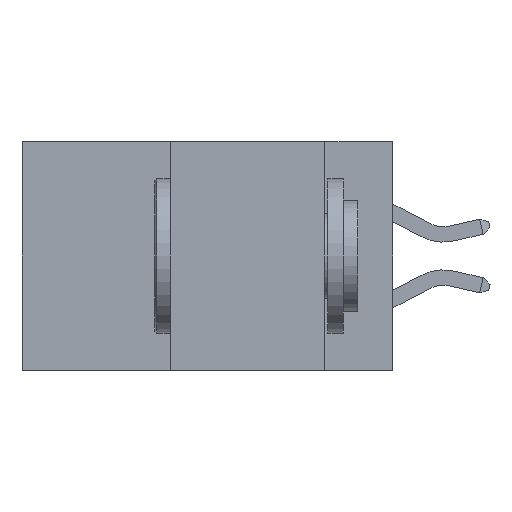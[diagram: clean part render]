
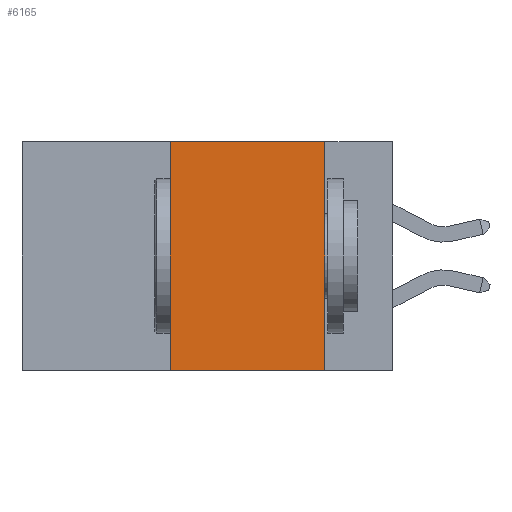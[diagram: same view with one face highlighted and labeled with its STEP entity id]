
A CAD part, left-side view. The second image highlights one B-rep face of the part: STEP entity #6165.
In plain terms, the highlighted planar face has unit normal (-1, 0, 0).
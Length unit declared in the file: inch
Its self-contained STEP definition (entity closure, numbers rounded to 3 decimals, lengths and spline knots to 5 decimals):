
#2321 = VERTEX_POINT ( 'NONE', #10326 ) ;
#2730 = AXIS2_PLACEMENT_3D ( 'NONE', #5660, #5352, #22209 ) ;
#3332 = CARTESIAN_POINT ( 'NONE',  ( 0., 0.11, 0. ) ) ;
#5352 = DIRECTION ( 'NONE',  ( 1., 0., 0. ) ) ;
#5660 = CARTESIAN_POINT ( 'NONE',  ( 0., 0.6, 0. ) ) ;
#6165 = ADVANCED_FACE ( 'NONE', ( #21445 ), #10330, .F. ) ;
#6452 = EDGE_CURVE ( 'NONE', #12743, #2321, #17380, .T. ) ;
#6535 = VERTEX_POINT ( 'NONE', #13450 ) ;
#8285 = EDGE_LOOP ( 'NONE', ( #12414, #28717, #10790, #28006 ) ) ;
#10326 = CARTESIAN_POINT ( 'NONE',  ( 0., 0.11, -0.37 ) ) ;
#10330 = PLANE ( 'NONE',  #2730 ) ;
#10790 = ORIENTED_EDGE ( 'NONE', *, *, #23180, .F. ) ;
#11080 = VECTOR ( 'NONE', #12048, 39.37008 ) ;
#12048 = DIRECTION ( 'NONE',  ( 0., -1., 0. ) ) ;
#12414 = ORIENTED_EDGE ( 'NONE', *, *, #20497, .F. ) ;
#12743 = VERTEX_POINT ( 'NONE', #20016 ) ;
#13012 = DIRECTION ( 'NONE',  ( 0., 0., -1. ) ) ;
#13141 = VERTEX_POINT ( 'NONE', #13917 ) ;
#13211 = DIRECTION ( 'NONE',  ( 0., -1., 0. ) ) ;
#13450 = CARTESIAN_POINT ( 'NONE',  ( 0., 0.11, 0. ) ) ;
#13466 = VECTOR ( 'NONE', #13012, 39.37008 ) ;
#13917 = CARTESIAN_POINT ( 'NONE',  ( 0., 0.36, 0. ) ) ;
#14044 = VECTOR ( 'NONE', #19720, 39.37008 ) ;
#17380 = LINE ( 'NONE', #18390, #11080 ) ;
#17430 = CARTESIAN_POINT ( 'NONE',  ( 0., 0.36, 0. ) ) ;
#18390 = CARTESIAN_POINT ( 'NONE',  ( 0., 0.6, -0.37 ) ) ;
#19720 = DIRECTION ( 'NONE',  ( 0., 0., 1. ) ) ;
#20016 = CARTESIAN_POINT ( 'NONE',  ( 0., 0.36, -0.37 ) ) ;
#20497 = EDGE_CURVE ( 'NONE', #6535, #2321, #24195, .T. ) ;
#20694 = EDGE_CURVE ( 'NONE', #13141, #6535, #23434, .T. ) ;
#21445 = FACE_OUTER_BOUND ( 'NONE', #8285, .T. ) ;
#22209 = DIRECTION ( 'NONE',  ( 0., 0., -1. ) ) ;
#23180 = EDGE_CURVE ( 'NONE', #12743, #13141, #23632, .T. ) ;
#23434 = LINE ( 'NONE', #30077, #27929 ) ;
#23632 = LINE ( 'NONE', #17430, #14044 ) ;
#24195 = LINE ( 'NONE', #3332, #13466 ) ;
#27929 = VECTOR ( 'NONE', #13211, 39.37008 ) ;
#28006 = ORIENTED_EDGE ( 'NONE', *, *, #6452, .T. ) ;
#28717 = ORIENTED_EDGE ( 'NONE', *, *, #20694, .F. ) ;
#30077 = CARTESIAN_POINT ( 'NONE',  ( 0., 0.6, 0. ) ) ;
